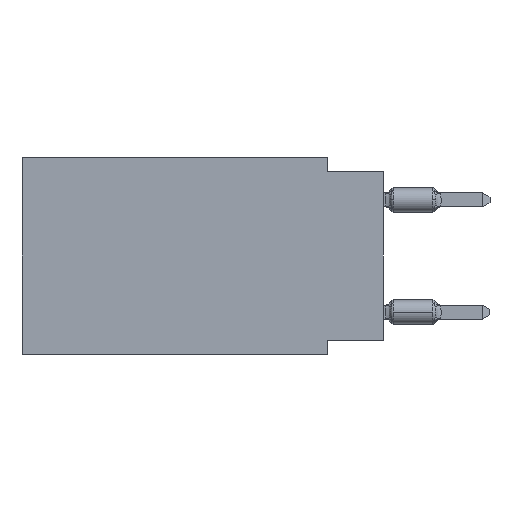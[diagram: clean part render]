
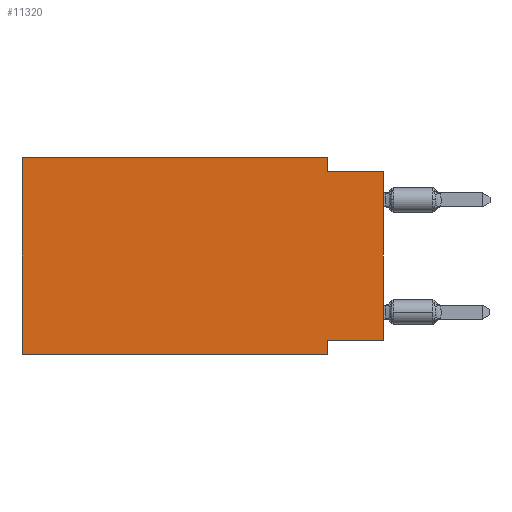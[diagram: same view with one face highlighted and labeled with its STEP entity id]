
A CAD part, left-side view. The second image highlights one B-rep face of the part: STEP entity #11320.
In plain terms, the highlighted planar face has unit normal (-1, 0, 0).
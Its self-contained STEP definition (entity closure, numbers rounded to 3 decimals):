
#205 = CARTESIAN_POINT ( 'NONE',  ( 0., 16.383, 0. ) ) ;
#292 = EDGE_CURVE ( 'NONE', #1275, #6954, #7800, .T. ) ;
#323 = DIRECTION ( 'NONE',  ( 0., 0., 1. ) ) ;
#428 = VERTEX_POINT ( 'NONE', #10555 ) ;
#704 = DIRECTION ( 'NONE',  ( 0., 0., 1. ) ) ;
#921 = DIRECTION ( 'NONE',  ( 0., 0., -1. ) ) ;
#958 = LINE ( 'NONE', #13885, #10710 ) ;
#1031 = ORIENTED_EDGE ( 'NONE', *, *, #292, .F. ) ;
#1120 = PLANE ( 'NONE',  #2096 ) ;
#1133 = VERTEX_POINT ( 'NONE', #6637 ) ;
#1275 = VERTEX_POINT ( 'NONE', #5605 ) ;
#1963 = ORIENTED_EDGE ( 'NONE', *, *, #9848, .F. ) ;
#2096 = AXIS2_PLACEMENT_3D ( 'NONE', #205, #2178, #2306 ) ;
#2098 = DIRECTION ( 'NONE',  ( 0., 1., 0. ) ) ;
#2178 = DIRECTION ( 'NONE',  ( 1., 0., 0. ) ) ;
#2274 = CARTESIAN_POINT ( 'NONE',  ( 0., 2.54, -8.89 ) ) ;
#2306 = DIRECTION ( 'NONE',  ( 0., 0., -1. ) ) ;
#2374 = EDGE_CURVE ( 'NONE', #6954, #12974, #958, .T. ) ;
#2511 = VERTEX_POINT ( 'NONE', #13582 ) ;
#2635 = ORIENTED_EDGE ( 'NONE', *, *, #2374, .F. ) ;
#2796 = VECTOR ( 'NONE', #4663, 1000. ) ;
#3164 = VECTOR ( 'NONE', #323, 1000. ) ;
#3993 = EDGE_CURVE ( 'NONE', #428, #4707, #5082, .T. ) ;
#4534 = DIRECTION ( 'NONE',  ( 0., 0., -1. ) ) ;
#4663 = DIRECTION ( 'NONE',  ( 0., -1., 0. ) ) ;
#4707 = VERTEX_POINT ( 'NONE', #8212 ) ;
#5082 = LINE ( 'NONE', #8317, #5708 ) ;
#5148 = CARTESIAN_POINT ( 'NONE',  ( 0., 2.54, 0. ) ) ;
#5474 = CARTESIAN_POINT ( 'NONE',  ( 0., 16.383, -8.89 ) ) ;
#5605 = CARTESIAN_POINT ( 'NONE',  ( 0., 16.383, -8.89 ) ) ;
#5708 = VECTOR ( 'NONE', #704, 1000. ) ;
#5728 = EDGE_CURVE ( 'NONE', #1275, #8963, #12830, .T. ) ;
#5998 = ORIENTED_EDGE ( 'NONE', *, *, #10596, .F. ) ;
#6331 = DIRECTION ( 'NONE',  ( 0., -1., 0. ) ) ;
#6583 = ORIENTED_EDGE ( 'NONE', *, *, #8488, .F. ) ;
#6637 = CARTESIAN_POINT ( 'NONE',  ( 0., 2.54, -8.255 ) ) ;
#6653 = ORIENTED_EDGE ( 'NONE', *, *, #5728, .T. ) ;
#6954 = VERTEX_POINT ( 'NONE', #11795 ) ;
#7401 = LINE ( 'NONE', #5148, #13432 ) ;
#7527 = CARTESIAN_POINT ( 'NONE',  ( 0., 2.54, 0. ) ) ;
#7741 = FACE_OUTER_BOUND ( 'NONE', #8505, .T. ) ;
#7800 = LINE ( 'NONE', #13164, #3164 ) ;
#8212 = CARTESIAN_POINT ( 'NONE',  ( 0., 0., -0.635 ) ) ;
#8224 = VECTOR ( 'NONE', #4534, 1000. ) ;
#8317 = CARTESIAN_POINT ( 'NONE',  ( 0., 0., 0. ) ) ;
#8488 = EDGE_CURVE ( 'NONE', #12974, #2511, #7401, .T. ) ;
#8505 = EDGE_LOOP ( 'NONE', ( #9905, #1963, #6583, #2635, #1031, #6653, #5998, #13793 ) ) ;
#8963 = VERTEX_POINT ( 'NONE', #11120 ) ;
#9114 = CARTESIAN_POINT ( 'NONE',  ( 0., 0., -0.635 ) ) ;
#9597 = VECTOR ( 'NONE', #6331, 1000. ) ;
#9848 = EDGE_CURVE ( 'NONE', #2511, #4707, #12223, .T. ) ;
#9905 = ORIENTED_EDGE ( 'NONE', *, *, #3993, .T. ) ;
#10555 = CARTESIAN_POINT ( 'NONE',  ( 0., 0., -8.255 ) ) ;
#10596 = EDGE_CURVE ( 'NONE', #1133, #8963, #11965, .T. ) ;
#10710 = VECTOR ( 'NONE', #12821, 1000. ) ;
#11109 = EDGE_CURVE ( 'NONE', #428, #1133, #13908, .T. ) ;
#11120 = CARTESIAN_POINT ( 'NONE',  ( 0., 2.54, -8.89 ) ) ;
#11320 = ADVANCED_FACE ( 'NONE', ( #7741 ), #1120, .F. ) ;
#11784 = CARTESIAN_POINT ( 'NONE',  ( 0., 0., -8.255 ) ) ;
#11795 = CARTESIAN_POINT ( 'NONE',  ( 0., 16.383, 0. ) ) ;
#11806 = VECTOR ( 'NONE', #2098, 1000. ) ;
#11965 = LINE ( 'NONE', #2274, #8224 ) ;
#12223 = LINE ( 'NONE', #9114, #2796 ) ;
#12821 = DIRECTION ( 'NONE',  ( 0., -1., 0. ) ) ;
#12830 = LINE ( 'NONE', #5474, #9597 ) ;
#12974 = VERTEX_POINT ( 'NONE', #7527 ) ;
#13164 = CARTESIAN_POINT ( 'NONE',  ( 0., 16.383, 0. ) ) ;
#13432 = VECTOR ( 'NONE', #921, 1000. ) ;
#13582 = CARTESIAN_POINT ( 'NONE',  ( 0., 2.54, -0.635 ) ) ;
#13793 = ORIENTED_EDGE ( 'NONE', *, *, #11109, .F. ) ;
#13885 = CARTESIAN_POINT ( 'NONE',  ( 0., 16.383, 0. ) ) ;
#13908 = LINE ( 'NONE', #11784, #11806 ) ;
